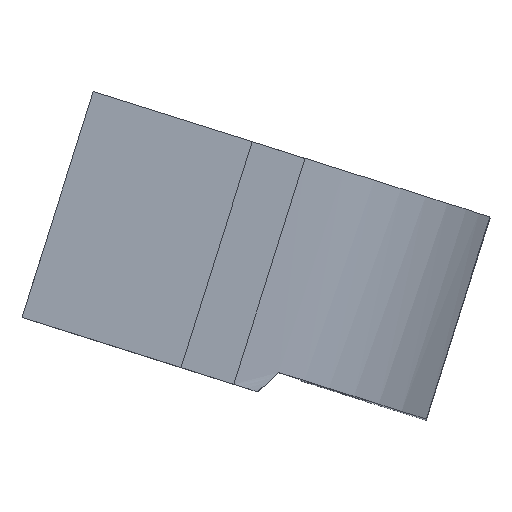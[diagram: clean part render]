
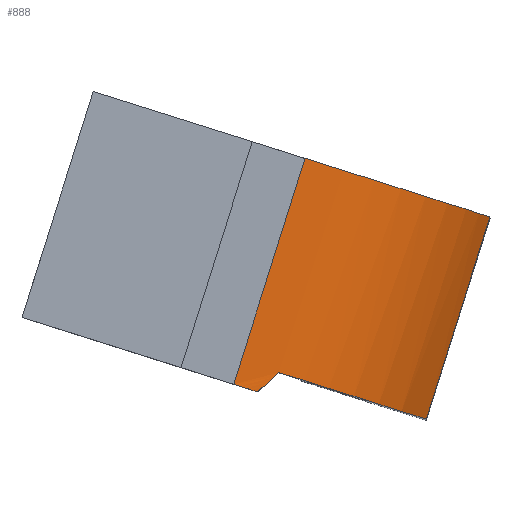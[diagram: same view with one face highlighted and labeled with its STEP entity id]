
A CAD part, top view. The second image highlights one B-rep face of the part: STEP entity #888.
In plain terms, the highlighted free-form (B-spline) face has degree [3, 1] with [13, 2] control points.
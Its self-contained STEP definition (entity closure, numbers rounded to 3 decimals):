
#15=ELLIPSE('',#963,34.462,14.358);
#16=ELLIPSE('',#964,16.029,9.8);
#17=B_SPLINE_SURFACE_WITH_KNOTS('',3,1,((#1372,#1373),(#1374,#1375),(#1376,
#1377),(#1378,#1379),(#1380,#1381),(#1382,#1383),(#1384,#1385),(#1386,#1387),
(#1388,#1389),(#1390,#1391),(#1392,#1393),(#1394,#1395),(#1396,#1397)),
 .UNSPECIFIED.,.F.,.F.,.F.,(4,1,1,1,1,1,1,1,1,1,4),(2,2),(0.01,
0.1,0.191,0.281,0.371,
0.462,0.559,0.666,0.788,
0.925,0.99),(0.,15.9),.UNSPECIFIED.);
#19=B_SPLINE_CURVE_WITH_KNOTS('',3,(#1332,#1333,#1334,#1335,#1336,#1337,
#1338,#1339,#1340,#1341,#1342,#1343),.UNSPECIFIED.,.F.,.F.,(4,1,1,1,1,1,
1,1,1,4),(0.01,0.075,0.212,0.334,
0.441,0.538,0.629,0.719,0.809,
0.831),.UNSPECIFIED.);
#21=B_SPLINE_CURVE_WITH_KNOTS('',3,(#1401,#1402,#1403,#1404,#1405,#1406,
#1407,#1408,#1409,#1410,#1411,#1412,#1413),.UNSPECIFIED.,.F.,.F.,(4,1,1,
1,1,1,1,1,1,1,4),(-0.99,-0.9,-0.809,-0.719,
-0.629,-0.538,-0.441,-0.334,-0.212,
-0.075,-0.01),.UNSPECIFIED.);
#70=FACE_OUTER_BOUND('',#117,.T.);
#117=EDGE_LOOP('',(#628,#629,#630,#631,#632,#633));
#164=LINE('',#1281,#263);
#186=LINE('',#1415,#285);
#263=VECTOR('',#1028,10.);
#285=VECTOR('',#1084,10.);
#359=VERTEX_POINT('',#1274);
#362=VERTEX_POINT('',#1279);
#386=VERTEX_POINT('',#1331);
#398=VERTEX_POINT('',#1398);
#399=VERTEX_POINT('',#1400);
#400=VERTEX_POINT('',#1414);
#452=EDGE_CURVE('',#362,#359,#164,.T.);
#477=EDGE_CURVE('',#359,#386,#19,.T.);
#490=EDGE_CURVE('',#386,#398,#15,.T.);
#491=EDGE_CURVE('',#399,#362,#21,.T.);
#492=EDGE_CURVE('',#400,#399,#186,.T.);
#493=EDGE_CURVE('',#398,#400,#16,.T.);
#628=ORIENTED_EDGE('',*,*,#490,.F.);
#629=ORIENTED_EDGE('',*,*,#477,.F.);
#630=ORIENTED_EDGE('',*,*,#452,.F.);
#631=ORIENTED_EDGE('',*,*,#491,.F.);
#632=ORIENTED_EDGE('',*,*,#492,.F.);
#633=ORIENTED_EDGE('',*,*,#493,.F.);
#888=ADVANCED_FACE('',(#70),#17,.T.);
#963=AXIS2_PLACEMENT_3D('',#1399,#1082,#1083);
#964=AXIS2_PLACEMENT_3D('',#1416,#1085,#1086);
#1028=DIRECTION('',(-0.301,-0.954,0.));
#1082=DIRECTION('center_axis',(0.676,-0.737,0.));
#1083=DIRECTION('ref_axis',(0.688,0.63,0.36));
#1084=DIRECTION('',(0.301,0.954,0.));
#1085=DIRECTION('center_axis',(-0.301,-0.954,0.));
#1086=DIRECTION('ref_axis',(-0.645,0.203,-0.737));
#1274=CARTESIAN_POINT('',(60.714,-41.631,9.854));
#1279=CARTESIAN_POINT('',(63.029,-34.288,9.854));
#1281=CARTESIAN_POINT('',(63.029,-34.288,9.854));
#1331=CARTESIAN_POINT('',(55.364,-39.944,14.289));
#1332=CARTESIAN_POINT('Ctrl Pts',(60.714,-41.631,9.854));
#1333=CARTESIAN_POINT('Ctrl Pts',(60.63,-41.605,10.032));
#1334=CARTESIAN_POINT('Ctrl Pts',(60.357,-41.519,10.573));
#1335=CARTESIAN_POINT('Ctrl Pts',(59.852,-41.359,11.4));
#1336=CARTESIAN_POINT('Ctrl Pts',(59.17,-41.144,12.248));
#1337=CARTESIAN_POINT('Ctrl Pts',(58.467,-40.923,12.906));
#1338=CARTESIAN_POINT('Ctrl Pts',(57.761,-40.7,13.408));
#1339=CARTESIAN_POINT('Ctrl Pts',(57.049,-40.476,13.791));
#1340=CARTESIAN_POINT('Ctrl Pts',(56.316,-40.244,14.076));
#1341=CARTESIAN_POINT('Ctrl Pts',(55.748,-40.065,14.22));
#1342=CARTESIAN_POINT('Ctrl Pts',(55.428,-39.965,14.278));
#1343=CARTESIAN_POINT('Ctrl Pts',(55.364,-39.944,14.289));
#1372=CARTESIAN_POINT('Ctrl Pts',(53.727,-40.372,14.4));
#1373=CARTESIAN_POINT('Ctrl Pts',(101.539,111.27,14.4));
#1374=CARTESIAN_POINT('Ctrl Pts',(53.987,-40.454,14.4));
#1375=CARTESIAN_POINT('Ctrl Pts',(101.799,111.188,14.4));
#1376=CARTESIAN_POINT('Ctrl Pts',(54.509,-40.618,14.377));
#1377=CARTESIAN_POINT('Ctrl Pts',(102.321,111.023,14.377));
#1378=CARTESIAN_POINT('Ctrl Pts',(55.285,-40.863,14.268));
#1379=CARTESIAN_POINT('Ctrl Pts',(103.098,110.778,14.268));
#1380=CARTESIAN_POINT('Ctrl Pts',(56.045,-41.103,14.076));
#1381=CARTESIAN_POINT('Ctrl Pts',(103.858,110.539,14.076));
#1382=CARTESIAN_POINT('Ctrl Pts',(56.778,-41.334,13.791));
#1383=CARTESIAN_POINT('Ctrl Pts',(104.591,110.307,13.791));
#1384=CARTESIAN_POINT('Ctrl Pts',(57.491,-41.559,13.408));
#1385=CARTESIAN_POINT('Ctrl Pts',(105.303,110.083,13.408));
#1386=CARTESIAN_POINT('Ctrl Pts',(58.197,-41.781,12.906));
#1387=CARTESIAN_POINT('Ctrl Pts',(106.009,109.86,12.906));
#1388=CARTESIAN_POINT('Ctrl Pts',(58.899,-42.003,12.248));
#1389=CARTESIAN_POINT('Ctrl Pts',(106.712,109.639,12.248));
#1390=CARTESIAN_POINT('Ctrl Pts',(59.581,-42.218,11.4));
#1391=CARTESIAN_POINT('Ctrl Pts',(107.394,109.424,11.4));
#1392=CARTESIAN_POINT('Ctrl Pts',(60.087,-42.377,10.573));
#1393=CARTESIAN_POINT('Ctrl Pts',(107.899,109.264,10.573));
#1394=CARTESIAN_POINT('Ctrl Pts',(60.359,-42.463,10.032));
#1395=CARTESIAN_POINT('Ctrl Pts',(108.172,109.178,10.032));
#1396=CARTESIAN_POINT('Ctrl Pts',(60.443,-42.49,9.854));
#1397=CARTESIAN_POINT('Ctrl Pts',(108.256,109.152,9.854));
#1398=CARTESIAN_POINT('',(54.598,-40.647,14.356));
#1399=CARTESIAN_POINT('Origin',(39.936,-54.084,-3.854));
#1400=CARTESIAN_POINT('',(56.313,-32.17,14.4));
#1401=CARTESIAN_POINT('Ctrl Pts',(56.313,-32.17,14.4));
#1402=CARTESIAN_POINT('Ctrl Pts',(56.573,-32.252,14.4));
#1403=CARTESIAN_POINT('Ctrl Pts',(57.095,-32.417,14.377));
#1404=CARTESIAN_POINT('Ctrl Pts',(57.872,-32.661,14.268));
#1405=CARTESIAN_POINT('Ctrl Pts',(58.631,-32.901,14.076));
#1406=CARTESIAN_POINT('Ctrl Pts',(59.364,-33.132,13.791));
#1407=CARTESIAN_POINT('Ctrl Pts',(60.077,-33.357,13.408));
#1408=CARTESIAN_POINT('Ctrl Pts',(60.783,-33.579,12.906));
#1409=CARTESIAN_POINT('Ctrl Pts',(61.485,-33.801,12.248));
#1410=CARTESIAN_POINT('Ctrl Pts',(62.167,-34.016,11.4));
#1411=CARTESIAN_POINT('Ctrl Pts',(62.673,-34.175,10.573));
#1412=CARTESIAN_POINT('Ctrl Pts',(62.945,-34.261,10.032));
#1413=CARTESIAN_POINT('Ctrl Pts',(63.029,-34.288,9.854));
#1414=CARTESIAN_POINT('',(53.727,-40.372,14.4));
#1415=CARTESIAN_POINT('',(53.727,-40.372,14.4));
#1416=CARTESIAN_POINT('Origin',(48.083,-38.592,0.857));
